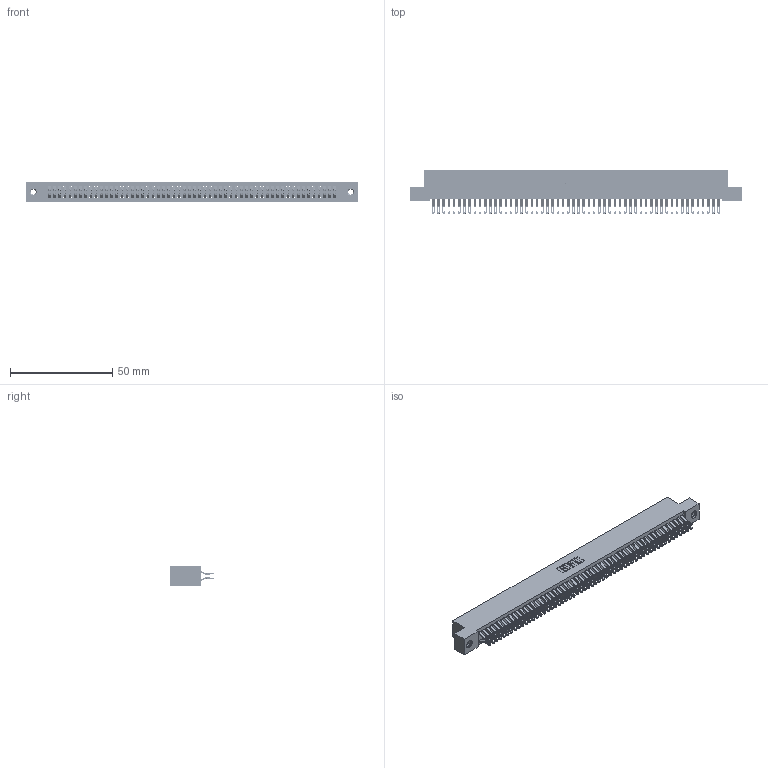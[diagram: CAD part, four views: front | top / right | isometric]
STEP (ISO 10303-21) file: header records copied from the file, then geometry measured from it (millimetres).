
FILE_DESCRIPTION (( 'STEP AP203' ), '1' );
FILE_NAME ('392-112-555-207.STEP', '2019-10-10T00:34:53', ( '' ), ( '' ), 'SwSTEP 2.0', 'SolidWorks 2016', '' );
FILE_SCHEMA (( 'CONFIG_CONTROL_DESIGN' ));
Length unit declared in the file: inch
Products named in the file (4): 342 Part_TI; 345-292-001_555 Tail; 345-250-001_345-250-005-103; 392-112-555-207
Assembly tree (115 placements, depth 2):
  392-112-555-207
    342 Part_TI
    345-292-001_555 Tail  x112
    345-250-001_345-250-005-103  x2
Bounding box: 162.56 x 21.47 x 9.4 mm (x, y, z)
Volume: 14970.8 mm3; surface area: 25823.2 mm2
Topology: 115 solids, 115 shells, 6666 faces, 20931 edges, 13946 vertices
Faces by surface type: plane 3906, cylinder 2744, cone 12, torus 4
Entity records: 35596 total; most frequent: CARTESIAN_POINT 5899, ORIENTED_EDGE 5798, DIRECTION 5017, EDGE_CURVE 2899, VECTOR 2731, LINE 2731, VERTEX_POINT 1928, AXIS2_PLACEMENT_3D 1143
